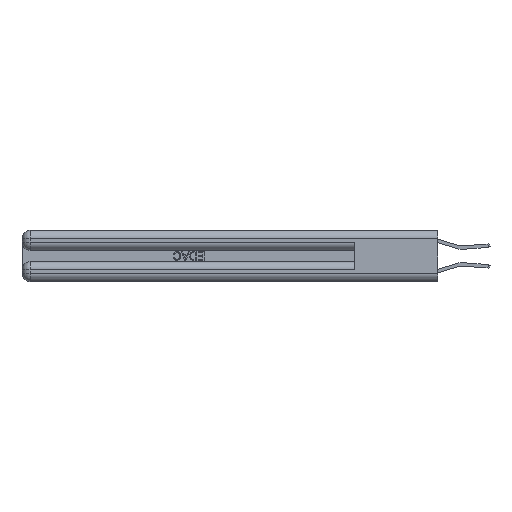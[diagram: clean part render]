
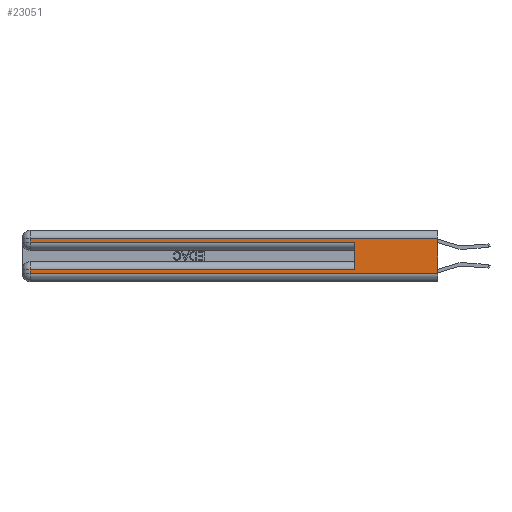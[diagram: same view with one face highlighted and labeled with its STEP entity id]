
A CAD part, left-side view. The second image highlights one B-rep face of the part: STEP entity #23051.
In plain terms, the highlighted planar face has unit normal (-1, 0, 0).
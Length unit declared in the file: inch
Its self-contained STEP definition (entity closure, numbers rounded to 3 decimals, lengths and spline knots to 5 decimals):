
#84 = EDGE_CURVE ( 'NONE', #6840, #8261, #16962, .T. ) ;
#149 = CARTESIAN_POINT ( 'NONE',  ( 0., 2.94, 0.06 ) ) ;
#593 = VECTOR ( 'NONE', #12193, 39.37008 ) ;
#1239 = ORIENTED_EDGE ( 'NONE', *, *, #2361, .T. ) ;
#1463 = CARTESIAN_POINT ( 'NONE',  ( 0., 0., 0.06 ) ) ;
#2361 = EDGE_CURVE ( 'NONE', #5261, #2792, #3581, .T. ) ;
#2684 = DIRECTION ( 'NONE',  ( 0., -1., 0. ) ) ;
#2792 = VERTEX_POINT ( 'NONE', #28325 ) ;
#2829 = VECTOR ( 'NONE', #14910, 39.37008 ) ;
#3337 = LINE ( 'NONE', #23573, #17597 ) ;
#3581 = LINE ( 'NONE', #27948, #11940 ) ;
#3936 = CARTESIAN_POINT ( 'NONE',  ( 0., 2.94, 0.085 ) ) ;
#3952 = CARTESIAN_POINT ( 'NONE',  ( 0., 0., 0.31 ) ) ;
#4102 = VECTOR ( 'NONE', #23811, 39.37008 ) ;
#4132 = LINE ( 'NONE', #14878, #4102 ) ;
#4600 = CARTESIAN_POINT ( 'NONE',  ( 0., 0.6, 0.285 ) ) ;
#5261 = VERTEX_POINT ( 'NONE', #8541 ) ;
#6840 = VERTEX_POINT ( 'NONE', #22607 ) ;
#7068 = LINE ( 'NONE', #13528, #9267 ) ;
#7608 = ORIENTED_EDGE ( 'NONE', *, *, #20858, .T. ) ;
#8261 = VERTEX_POINT ( 'NONE', #3936 ) ;
#8541 = CARTESIAN_POINT ( 'NONE',  ( 0., 2.94, 0.31 ) ) ;
#8899 = ORIENTED_EDGE ( 'NONE', *, *, #17998, .F. ) ;
#9255 = DIRECTION ( 'NONE',  ( 0., -1., 0. ) ) ;
#9267 = VECTOR ( 'NONE', #27147, 39.37008 ) ;
#9429 = PLANE ( 'NONE',  #16764 ) ;
#9595 = LINE ( 'NONE', #24856, #24622 ) ;
#10221 = CARTESIAN_POINT ( 'NONE',  ( 0., 0., 0.085 ) ) ;
#10270 = CARTESIAN_POINT ( 'NONE',  ( 0., 0.6, 0.145 ) ) ;
#10284 = VECTOR ( 'NONE', #9255, 39.37008 ) ;
#11188 = CARTESIAN_POINT ( 'NONE',  ( 0., 0., 0.06 ) ) ;
#11199 = VERTEX_POINT ( 'NONE', #149 ) ;
#11940 = VECTOR ( 'NONE', #28089, 39.37008 ) ;
#12193 = DIRECTION ( 'NONE',  ( 0., 0., 1. ) ) ;
#12463 = EDGE_CURVE ( 'NONE', #16245, #24983, #3337, .T. ) ;
#12784 = ORIENTED_EDGE ( 'NONE', *, *, #84, .T. ) ;
#13528 = CARTESIAN_POINT ( 'NONE',  ( 0., 0., 0.31 ) ) ;
#14878 = CARTESIAN_POINT ( 'NONE',  ( 0., 2.94, 0.37 ) ) ;
#14910 = DIRECTION ( 'NONE',  ( 0., 1., 0. ) ) ;
#14953 = LINE ( 'NONE', #10270, #593 ) ;
#16245 = VERTEX_POINT ( 'NONE', #3952 ) ;
#16764 = AXIS2_PLACEMENT_3D ( 'NONE', #18393, #24540, #20311 ) ;
#16962 = LINE ( 'NONE', #10221, #2829 ) ;
#17051 = ORIENTED_EDGE ( 'NONE', *, *, #12463, .F. ) ;
#17597 = VECTOR ( 'NONE', #23297, 39.37008 ) ;
#17832 = FACE_OUTER_BOUND ( 'NONE', #18105, .T. ) ;
#17998 = EDGE_CURVE ( 'NONE', #6840, #25702, #14953, .T. ) ;
#18105 = EDGE_LOOP ( 'NONE', ( #17051, #21828, #1239, #24182, #8899, #12784, #7608, #18872 ) ) ;
#18393 = CARTESIAN_POINT ( 'NONE',  ( 0., 0., 0.37 ) ) ;
#18872 = ORIENTED_EDGE ( 'NONE', *, *, #24721, .T. ) ;
#20015 = LINE ( 'NONE', #11188, #10284 ) ;
#20311 = DIRECTION ( 'NONE',  ( 0., 0., -1. ) ) ;
#20858 = EDGE_CURVE ( 'NONE', #8261, #11199, #4132, .T. ) ;
#21828 = ORIENTED_EDGE ( 'NONE', *, *, #23544, .T. ) ;
#22607 = CARTESIAN_POINT ( 'NONE',  ( 0., 0.6, 0.085 ) ) ;
#23051 = ADVANCED_FACE ( 'NONE', ( #17832 ), #9429, .F. ) ;
#23297 = DIRECTION ( 'NONE',  ( 0., 0., -1. ) ) ;
#23544 = EDGE_CURVE ( 'NONE', #16245, #5261, #7068, .T. ) ;
#23573 = CARTESIAN_POINT ( 'NONE',  ( 0., 0., 0.37 ) ) ;
#23811 = DIRECTION ( 'NONE',  ( 0., 0., -1. ) ) ;
#24182 = ORIENTED_EDGE ( 'NONE', *, *, #25594, .T. ) ;
#24540 = DIRECTION ( 'NONE',  ( 1., 0., 0. ) ) ;
#24622 = VECTOR ( 'NONE', #2684, 39.37008 ) ;
#24721 = EDGE_CURVE ( 'NONE', #11199, #24983, #20015, .T. ) ;
#24856 = CARTESIAN_POINT ( 'NONE',  ( 0., 0., 0.285 ) ) ;
#24983 = VERTEX_POINT ( 'NONE', #1463 ) ;
#25594 = EDGE_CURVE ( 'NONE', #2792, #25702, #9595, .T. ) ;
#25702 = VERTEX_POINT ( 'NONE', #4600 ) ;
#27147 = DIRECTION ( 'NONE',  ( 0., 1., 0. ) ) ;
#27948 = CARTESIAN_POINT ( 'NONE',  ( 0., 2.94, 0.37 ) ) ;
#28089 = DIRECTION ( 'NONE',  ( 0., 0., -1. ) ) ;
#28325 = CARTESIAN_POINT ( 'NONE',  ( 0., 2.94, 0.285 ) ) ;
